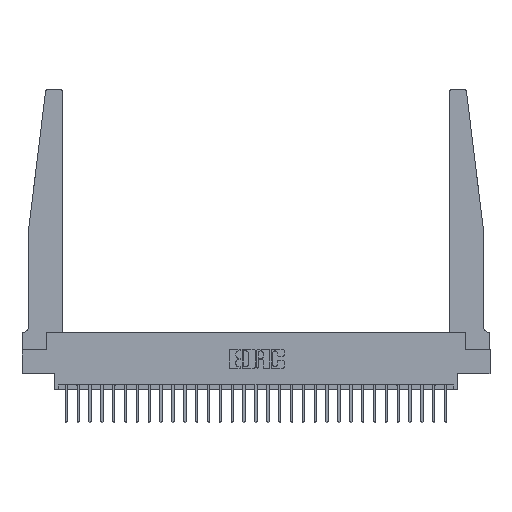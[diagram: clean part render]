
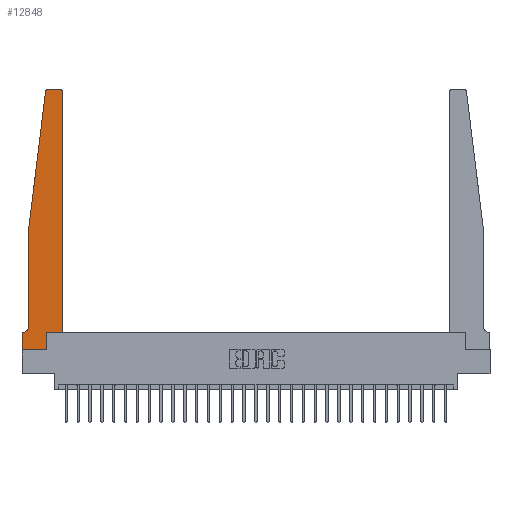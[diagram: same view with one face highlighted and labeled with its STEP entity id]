
A CAD part, top view. The second image highlights one B-rep face of the part: STEP entity #12848.
In plain terms, the highlighted planar face has unit normal (0, 0, 1).
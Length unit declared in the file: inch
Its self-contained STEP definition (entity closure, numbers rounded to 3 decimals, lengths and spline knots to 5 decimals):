
#492 = AXIS2_PLACEMENT_3D ( 'NONE', #4496, #19433, #6704 ) ;
#685 = LINE ( 'NONE', #22945, #22140 ) ;
#1082 = EDGE_CURVE ( 'NONE', #9096, #17141, #6957, .T. ) ;
#1379 = LINE ( 'NONE', #22610, #7240 ) ;
#1471 = ORIENTED_EDGE ( 'NONE', *, *, #26072, .T. ) ;
#3273 = VERTEX_POINT ( 'NONE', #11048 ) ;
#3544 = EDGE_CURVE ( 'NONE', #13307, #3273, #1379, .T. ) ;
#4397 = EDGE_CURVE ( 'NONE', #17012, #9791, #685, .T. ) ;
#4496 = CARTESIAN_POINT ( 'NONE',  ( 0.015, 0.2375, 0.37 ) ) ;
#4523 = LINE ( 'NONE', #12200, #15239 ) ;
#4713 = CARTESIAN_POINT ( 'NONE',  ( 0.27653, 2.75, 0.37 ) ) ;
#4815 = EDGE_LOOP ( 'NONE', ( #17275, #25594, #8443, #22339, #24062, #27357, #20168, #16390, #20908, #1471, #12486, #20351 ) ) ;
#5042 = LINE ( 'NONE', #6261, #17078 ) ;
#5145 = DIRECTION ( 'NONE',  ( 1., 0., 0. ) ) ;
#5374 = CARTESIAN_POINT ( 'NONE',  ( 0.425, 0.18, 0.37 ) ) ;
#5657 = DIRECTION ( 'NONE',  ( -1., 0., 0. ) ) ;
#6261 = CARTESIAN_POINT ( 'NONE',  ( 0.065, 1.25, 0.37 ) ) ;
#6335 = CARTESIAN_POINT ( 'NONE',  ( 0., 0., 0.37 ) ) ;
#6704 = DIRECTION ( 'NONE',  ( -1., 0., 0. ) ) ;
#6816 = CARTESIAN_POINT ( 'NONE',  ( 0.065, 1.25, 0.37 ) ) ;
#6957 = LINE ( 'NONE', #6335, #17607 ) ;
#7240 = VECTOR ( 'NONE', #24732, 39.37008 ) ;
#7746 = FACE_OUTER_BOUND ( 'NONE', #4815, .T. ) ;
#8126 = DIRECTION ( 'NONE',  ( 0., 1., 0. ) ) ;
#8443 = ORIENTED_EDGE ( 'NONE', *, *, #18020, .T. ) ;
#8797 = CARTESIAN_POINT ( 'NONE',  ( 0.065, 1.25, 0.37 ) ) ;
#9096 = VERTEX_POINT ( 'NONE', #13678 ) ;
#9433 = CARTESIAN_POINT ( 'NONE',  ( 0.015, 0.1875, 0.37 ) ) ;
#9449 = LINE ( 'NONE', #23426, #14484 ) ;
#9791 = VERTEX_POINT ( 'NONE', #26823 ) ;
#10284 = LINE ( 'NONE', #14150, #15323 ) ;
#10417 = CARTESIAN_POINT ( 'NONE',  ( 0., 0.1875, 0.37 ) ) ;
#10615 = DIRECTION ( 'NONE',  ( 0., 0., 1. ) ) ;
#10729 = CARTESIAN_POINT ( 'NONE',  ( 0.27653, 2.72, 0.37 ) ) ;
#10923 = CARTESIAN_POINT ( 'NONE',  ( 0.065, 0.2375, 0.37 ) ) ;
#11048 = CARTESIAN_POINT ( 'NONE',  ( 0.425, 2.72, 0.37 ) ) ;
#11595 = AXIS2_PLACEMENT_3D ( 'NONE', #10729, #25534, #12884 ) ;
#12059 = VERTEX_POINT ( 'NONE', #13754 ) ;
#12200 = CARTESIAN_POINT ( 'NONE',  ( 0.065, 0.1875, 0.37 ) ) ;
#12486 = ORIENTED_EDGE ( 'NONE', *, *, #3544, .T. ) ;
#12848 = ADVANCED_FACE ( 'NONE', ( #7746 ), #25233, .T. ) ;
#12876 = DIRECTION ( 'NONE',  ( 1., 0., 0. ) ) ;
#12884 = DIRECTION ( 'NONE',  ( 1., 0., 0. ) ) ;
#12987 = DIRECTION ( 'NONE',  ( -0.122, -0.992, 0. ) ) ;
#13100 = LINE ( 'NONE', #8797, #16787 ) ;
#13281 = CARTESIAN_POINT ( 'NONE',  ( 0.2605, 0., 0.37 ) ) ;
#13307 = VERTEX_POINT ( 'NONE', #5374 ) ;
#13678 = CARTESIAN_POINT ( 'NONE',  ( 0., 0.1875, 0.37 ) ) ;
#13754 = CARTESIAN_POINT ( 'NONE',  ( 0.24675, 2.72367, 0.37 ) ) ;
#14150 = CARTESIAN_POINT ( 'NONE',  ( 0.25, 2.75, 0.37 ) ) ;
#14306 = CIRCLE ( 'NONE', #492, 0.05 ) ;
#14371 = DIRECTION ( 'NONE',  ( -1., 0., 0. ) ) ;
#14484 = VECTOR ( 'NONE', #12876, 39.37008 ) ;
#14730 = DIRECTION ( 'NONE',  ( 1., 0., 0. ) ) ;
#15024 = EDGE_CURVE ( 'NONE', #21363, #15149, #14306, .T. ) ;
#15149 = VERTEX_POINT ( 'NONE', #9433 ) ;
#15239 = VECTOR ( 'NONE', #14371, 39.37008 ) ;
#15323 = VECTOR ( 'NONE', #5657, 39.37008 ) ;
#15803 = CARTESIAN_POINT ( 'NONE',  ( 0., 0., 0.37 ) ) ;
#16093 = CARTESIAN_POINT ( 'NONE',  ( 0., 0., 0.37 ) ) ;
#16390 = ORIENTED_EDGE ( 'NONE', *, *, #21549, .T. ) ;
#16392 = VERTEX_POINT ( 'NONE', #4713 ) ;
#16787 = VECTOR ( 'NONE', #12987, 39.37008 ) ;
#16790 = CIRCLE ( 'NONE', #17899, 0.03 ) ;
#17012 = VERTEX_POINT ( 'NONE', #13281 ) ;
#17078 = VECTOR ( 'NONE', #21104, 39.37008 ) ;
#17141 = VERTEX_POINT ( 'NONE', #16093 ) ;
#17275 = ORIENTED_EDGE ( 'NONE', *, *, #21011, .T. ) ;
#17607 = VECTOR ( 'NONE', #23272, 39.37008 ) ;
#17899 = AXIS2_PLACEMENT_3D ( 'NONE', #23319, #10615, #25433 ) ;
#18020 = EDGE_CURVE ( 'NONE', #12059, #23573, #13100, .T. ) ;
#19254 = CIRCLE ( 'NONE', #11595, 0.03 ) ;
#19433 = DIRECTION ( 'NONE',  ( 0., 0., -1. ) ) ;
#19598 = LINE ( 'NONE', #15803, #24509 ) ;
#20168 = ORIENTED_EDGE ( 'NONE', *, *, #1082, .T. ) ;
#20351 = ORIENTED_EDGE ( 'NONE', *, *, #26714, .T. ) ;
#20908 = ORIENTED_EDGE ( 'NONE', *, *, #4397, .T. ) ;
#20966 = VERTEX_POINT ( 'NONE', #26686 ) ;
#21011 = EDGE_CURVE ( 'NONE', #20966, #16392, #10284, .T. ) ;
#21104 = DIRECTION ( 'NONE',  ( 0., -1., 0. ) ) ;
#21363 = VERTEX_POINT ( 'NONE', #10923 ) ;
#21493 = AXIS2_PLACEMENT_3D ( 'NONE', #10417, #27360, #14730 ) ;
#21549 = EDGE_CURVE ( 'NONE', #17141, #17012, #19598, .T. ) ;
#22140 = VECTOR ( 'NONE', #8126, 39.37008 ) ;
#22339 = ORIENTED_EDGE ( 'NONE', *, *, #27418, .T. ) ;
#22610 = CARTESIAN_POINT ( 'NONE',  ( 0.425, 0.18, 0.37 ) ) ;
#22945 = CARTESIAN_POINT ( 'NONE',  ( 0.2605, 0.18, 0.37 ) ) ;
#23272 = DIRECTION ( 'NONE',  ( 0., -1., 0. ) ) ;
#23319 = CARTESIAN_POINT ( 'NONE',  ( 0.395, 2.72, 0.37 ) ) ;
#23426 = CARTESIAN_POINT ( 'NONE',  ( 0.425, 0.18, 0.37 ) ) ;
#23573 = VERTEX_POINT ( 'NONE', #6816 ) ;
#24062 = ORIENTED_EDGE ( 'NONE', *, *, #15024, .T. ) ;
#24126 = EDGE_CURVE ( 'NONE', #16392, #12059, #19254, .T. ) ;
#24509 = VECTOR ( 'NONE', #5145, 39.37008 ) ;
#24656 = EDGE_CURVE ( 'NONE', #15149, #9096, #4523, .T. ) ;
#24732 = DIRECTION ( 'NONE',  ( 0., 1., 0. ) ) ;
#25233 = PLANE ( 'NONE',  #21493 ) ;
#25433 = DIRECTION ( 'NONE',  ( 1., 0., 0. ) ) ;
#25534 = DIRECTION ( 'NONE',  ( 0., 0., 1. ) ) ;
#25594 = ORIENTED_EDGE ( 'NONE', *, *, #24126, .T. ) ;
#26072 = EDGE_CURVE ( 'NONE', #9791, #13307, #9449, .T. ) ;
#26686 = CARTESIAN_POINT ( 'NONE',  ( 0.395, 2.75, 0.37 ) ) ;
#26714 = EDGE_CURVE ( 'NONE', #3273, #20966, #16790, .T. ) ;
#26823 = CARTESIAN_POINT ( 'NONE',  ( 0.2605, 0.18, 0.37 ) ) ;
#27357 = ORIENTED_EDGE ( 'NONE', *, *, #24656, .T. ) ;
#27360 = DIRECTION ( 'NONE',  ( 0., 0., 1. ) ) ;
#27418 = EDGE_CURVE ( 'NONE', #23573, #21363, #5042, .T. ) ;
